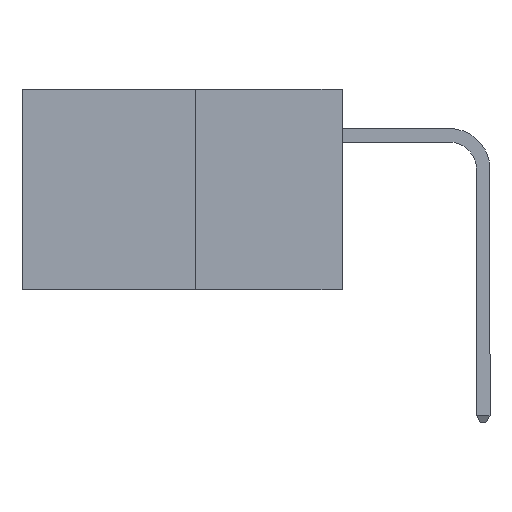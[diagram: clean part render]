
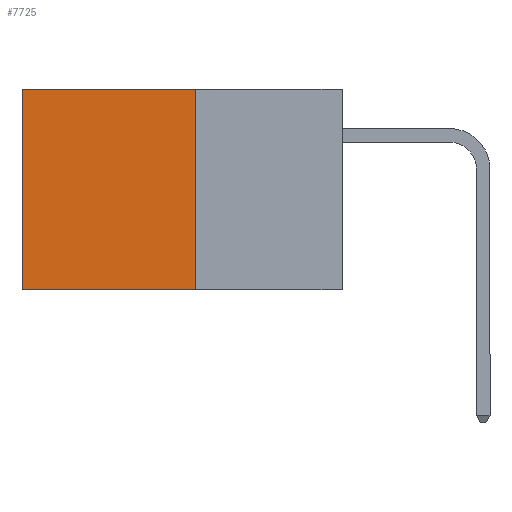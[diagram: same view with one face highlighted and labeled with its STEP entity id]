
A CAD part, left-side view. The second image highlights one B-rep face of the part: STEP entity #7725.
In plain terms, the highlighted planar face has unit normal (-1, 0, 0).
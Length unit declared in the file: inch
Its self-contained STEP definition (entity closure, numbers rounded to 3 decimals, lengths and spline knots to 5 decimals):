
#821 = CARTESIAN_POINT ( 'NONE',  ( 0.277, 0.59, 0. ) ) ;
#992 = VERTEX_POINT ( 'NONE', #821 ) ;
#1321 = PLANE ( 'NONE',  #18212 ) ;
#1636 = CARTESIAN_POINT ( 'NONE',  ( 0.277, 0.27, 0. ) ) ;
#1929 = EDGE_CURVE ( 'NONE', #26004, #992, #10882, .T. ) ;
#2223 = EDGE_CURVE ( 'NONE', #10915, #12433, #19805, .T. ) ;
#3190 = VECTOR ( 'NONE', #7321, 39.37008 ) ;
#4588 = VECTOR ( 'NONE', #17159, 39.37008 ) ;
#5559 = CARTESIAN_POINT ( 'NONE',  ( 0.277, 0.27, 0. ) ) ;
#5617 = CARTESIAN_POINT ( 'NONE',  ( 0.277, 0.27, -0.37 ) ) ;
#6630 = EDGE_CURVE ( 'NONE', #992, #12433, #10307, .T. ) ;
#7321 = DIRECTION ( 'NONE',  ( 0., 1., 0. ) ) ;
#7725 = ADVANCED_FACE ( 'NONE', ( #16882 ), #1321, .F. ) ;
#8783 = CARTESIAN_POINT ( 'NONE',  ( 0.277, 0.27, -0.37 ) ) ;
#10215 = VECTOR ( 'NONE', #16201, 39.37008 ) ;
#10307 = LINE ( 'NONE', #12845, #4588 ) ;
#10882 = LINE ( 'NONE', #5559, #10215 ) ;
#10894 = DIRECTION ( 'NONE',  ( 0., 0., -1. ) ) ;
#10915 = VERTEX_POINT ( 'NONE', #27237 ) ;
#11172 = CARTESIAN_POINT ( 'NONE',  ( 0.277, 0.59, -0.37 ) ) ;
#12124 = DIRECTION ( 'NONE',  ( 1., 0., 0. ) ) ;
#12433 = VERTEX_POINT ( 'NONE', #11172 ) ;
#12845 = CARTESIAN_POINT ( 'NONE',  ( 0.277, 0.59, -0.37 ) ) ;
#12876 = ORIENTED_EDGE ( 'NONE', *, *, #1929, .T. ) ;
#14083 = ORIENTED_EDGE ( 'NONE', *, *, #19979, .F. ) ;
#15402 = LINE ( 'NONE', #8783, #26053 ) ;
#16188 = EDGE_LOOP ( 'NONE', ( #27091, #21199, #14083, #12876 ) ) ;
#16201 = DIRECTION ( 'NONE',  ( 0., 1., 0. ) ) ;
#16882 = FACE_OUTER_BOUND ( 'NONE', #16188, .T. ) ;
#17159 = DIRECTION ( 'NONE',  ( 0., 0., -1. ) ) ;
#18212 = AXIS2_PLACEMENT_3D ( 'NONE', #24848, #12124, #26983 ) ;
#19805 = LINE ( 'NONE', #5617, #3190 ) ;
#19979 = EDGE_CURVE ( 'NONE', #26004, #10915, #15402, .T. ) ;
#21199 = ORIENTED_EDGE ( 'NONE', *, *, #2223, .F. ) ;
#24848 = CARTESIAN_POINT ( 'NONE',  ( 0.277, 0.27, -0.37 ) ) ;
#26004 = VERTEX_POINT ( 'NONE', #1636 ) ;
#26053 = VECTOR ( 'NONE', #10894, 39.37008 ) ;
#26983 = DIRECTION ( 'NONE',  ( 0., 0., -1. ) ) ;
#27091 = ORIENTED_EDGE ( 'NONE', *, *, #6630, .T. ) ;
#27237 = CARTESIAN_POINT ( 'NONE',  ( 0.277, 0.27, -0.37 ) ) ;
